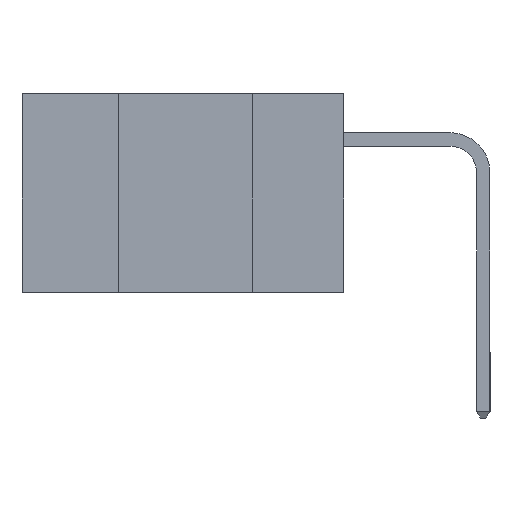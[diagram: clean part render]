
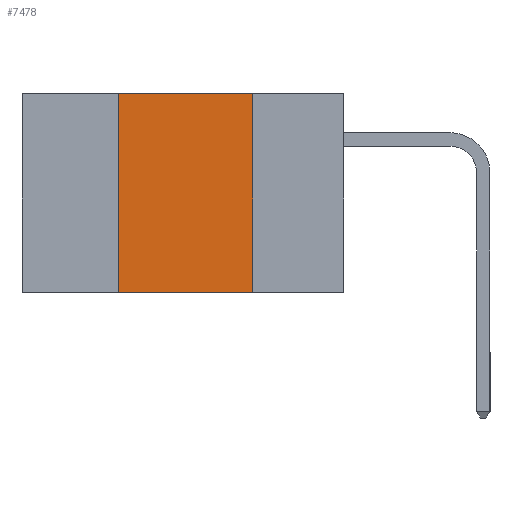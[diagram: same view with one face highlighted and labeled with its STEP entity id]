
A CAD part, left-side view. The second image highlights one B-rep face of the part: STEP entity #7478.
In plain terms, the highlighted planar face has unit normal (-1, 0, 0).
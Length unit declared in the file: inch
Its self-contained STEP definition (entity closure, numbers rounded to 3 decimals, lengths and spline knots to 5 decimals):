
#153 = CARTESIAN_POINT ( 'NONE',  ( 0., 0.6, 0. ) ) ;
#1012 = EDGE_CURVE ( 'NONE', #3824, #5706, #5720, .T. ) ;
#1104 = LINE ( 'NONE', #2704, #18794 ) ;
#1854 = ORIENTED_EDGE ( 'NONE', *, *, #1012, .F. ) ;
#2704 = CARTESIAN_POINT ( 'NONE',  ( 0., 0.42, 0. ) ) ;
#3824 = VERTEX_POINT ( 'NONE', #4659 ) ;
#4188 = CARTESIAN_POINT ( 'NONE',  ( 0., 0.42, -0.37 ) ) ;
#4209 = DIRECTION ( 'NONE',  ( 0., 0., 1. ) ) ;
#4659 = CARTESIAN_POINT ( 'NONE',  ( 0., 0.17, 0. ) ) ;
#5121 = DIRECTION ( 'NONE',  ( 0., 0., -1. ) ) ;
#5706 = VERTEX_POINT ( 'NONE', #7979 ) ;
#5720 = LINE ( 'NONE', #13757, #17530 ) ;
#5941 = DIRECTION ( 'NONE',  ( 0., -1., 0. ) ) ;
#5977 = VECTOR ( 'NONE', #5941, 39.37008 ) ;
#6973 = ORIENTED_EDGE ( 'NONE', *, *, #21437, .F. ) ;
#7332 = AXIS2_PLACEMENT_3D ( 'NONE', #153, #20847, #13826 ) ;
#7478 = ADVANCED_FACE ( 'NONE', ( #21029 ), #17253, .F. ) ;
#7979 = CARTESIAN_POINT ( 'NONE',  ( 0., 0.17, -0.37 ) ) ;
#8154 = ORIENTED_EDGE ( 'NONE', *, *, #20569, .T. ) ;
#10620 = VERTEX_POINT ( 'NONE', #21919 ) ;
#12086 = EDGE_LOOP ( 'NONE', ( #1854, #17634, #6973, #8154 ) ) ;
#13753 = DIRECTION ( 'NONE',  ( 0., -1., 0. ) ) ;
#13757 = CARTESIAN_POINT ( 'NONE',  ( 0., 0.17, 0. ) ) ;
#13826 = DIRECTION ( 'NONE',  ( 0., 0., -1. ) ) ;
#13886 = CARTESIAN_POINT ( 'NONE',  ( 0., 0.6, -0.37 ) ) ;
#15793 = LINE ( 'NONE', #13886, #17911 ) ;
#15955 = EDGE_CURVE ( 'NONE', #10620, #3824, #20455, .T. ) ;
#16210 = CARTESIAN_POINT ( 'NONE',  ( 0., 0.6, 0. ) ) ;
#17253 = PLANE ( 'NONE',  #7332 ) ;
#17530 = VECTOR ( 'NONE', #5121, 39.37008 ) ;
#17634 = ORIENTED_EDGE ( 'NONE', *, *, #15955, .F. ) ;
#17911 = VECTOR ( 'NONE', #13753, 39.37008 ) ;
#18794 = VECTOR ( 'NONE', #4209, 39.37008 ) ;
#20455 = LINE ( 'NONE', #16210, #5977 ) ;
#20569 = EDGE_CURVE ( 'NONE', #22016, #5706, #15793, .T. ) ;
#20847 = DIRECTION ( 'NONE',  ( 1., 0., 0. ) ) ;
#21029 = FACE_OUTER_BOUND ( 'NONE', #12086, .T. ) ;
#21437 = EDGE_CURVE ( 'NONE', #22016, #10620, #1104, .T. ) ;
#21919 = CARTESIAN_POINT ( 'NONE',  ( 0., 0.42, 0. ) ) ;
#22016 = VERTEX_POINT ( 'NONE', #4188 ) ;
